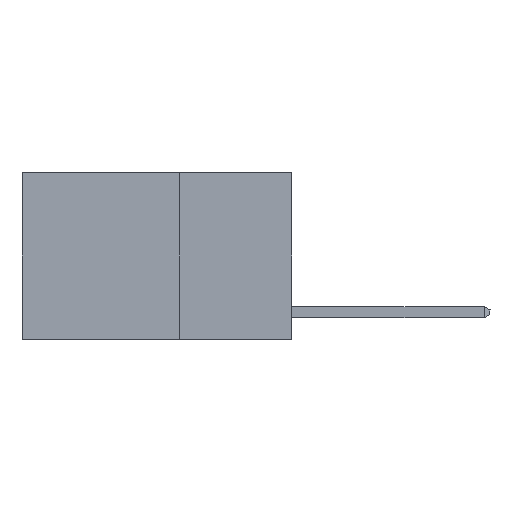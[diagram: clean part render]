
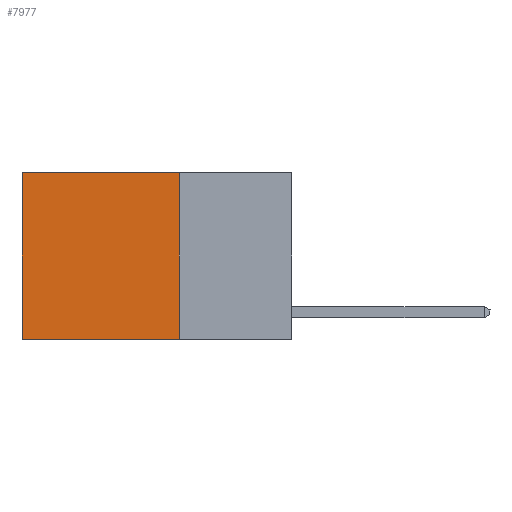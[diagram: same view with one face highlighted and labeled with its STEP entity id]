
A CAD part, left-side view. The second image highlights one B-rep face of the part: STEP entity #7977.
In plain terms, the highlighted planar face has unit normal (-1, 0, 0).
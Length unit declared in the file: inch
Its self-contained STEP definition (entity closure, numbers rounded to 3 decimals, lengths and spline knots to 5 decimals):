
#312 = LINE ( 'NONE', #19547, #20557 ) ;
#1221 = VERTEX_POINT ( 'NONE', #10538 ) ;
#2257 = LINE ( 'NONE', #14778, #7139 ) ;
#2525 = PLANE ( 'NONE',  #7700 ) ;
#3146 = CARTESIAN_POINT ( 'NONE',  ( 0.2625, 0.6, 0. ) ) ;
#3220 = DIRECTION ( 'NONE',  ( 0., 0., -1. ) ) ;
#3343 = DIRECTION ( 'NONE',  ( 0., 0., -1. ) ) ;
#5837 = DIRECTION ( 'NONE',  ( 0., 0., -1. ) ) ;
#6617 = CARTESIAN_POINT ( 'NONE',  ( 0.2625, 0.25, 0. ) ) ;
#7135 = VERTEX_POINT ( 'NONE', #11772 ) ;
#7139 = VECTOR ( 'NONE', #3343, 39.37008 ) ;
#7265 = DIRECTION ( 'NONE',  ( 0., 1., 0. ) ) ;
#7700 = AXIS2_PLACEMENT_3D ( 'NONE', #13976, #15629, #5837 ) ;
#7977 = ADVANCED_FACE ( 'NONE', ( #11208 ), #2525, .F. ) ;
#9650 = CARTESIAN_POINT ( 'NONE',  ( 0.2625, 0.25, -0.37 ) ) ;
#9879 = EDGE_CURVE ( 'NONE', #1221, #7135, #12168, .T. ) ;
#10538 = CARTESIAN_POINT ( 'NONE',  ( 0.2625, 0.25, -0.37 ) ) ;
#11208 = FACE_OUTER_BOUND ( 'NONE', #18272, .T. ) ;
#11658 = VECTOR ( 'NONE', #14513, 39.37008 ) ;
#11772 = CARTESIAN_POINT ( 'NONE',  ( 0.2625, 0.6, -0.37 ) ) ;
#12168 = LINE ( 'NONE', #9650, #11658 ) ;
#12485 = ORIENTED_EDGE ( 'NONE', *, *, #19044, .T. ) ;
#12974 = LINE ( 'NONE', #17092, #17347 ) ;
#13976 = CARTESIAN_POINT ( 'NONE',  ( 0.2625, 0.25, 0. ) ) ;
#14500 = VERTEX_POINT ( 'NONE', #6617 ) ;
#14513 = DIRECTION ( 'NONE',  ( 0., 1., 0. ) ) ;
#14778 = CARTESIAN_POINT ( 'NONE',  ( 0.2625, 0.6, 0. ) ) ;
#15321 = VERTEX_POINT ( 'NONE', #3146 ) ;
#15340 = EDGE_CURVE ( 'NONE', #14500, #1221, #312, .T. ) ;
#15629 = DIRECTION ( 'NONE',  ( 1., 0., 0. ) ) ;
#16818 = ORIENTED_EDGE ( 'NONE', *, *, #15340, .F. ) ;
#17092 = CARTESIAN_POINT ( 'NONE',  ( 0.2625, 0.25, 0. ) ) ;
#17347 = VECTOR ( 'NONE', #7265, 39.37008 ) ;
#17406 = ORIENTED_EDGE ( 'NONE', *, *, #17868, .T. ) ;
#17868 = EDGE_CURVE ( 'NONE', #15321, #7135, #2257, .T. ) ;
#18272 = EDGE_LOOP ( 'NONE', ( #17406, #19091, #16818, #12485 ) ) ;
#19044 = EDGE_CURVE ( 'NONE', #14500, #15321, #12974, .T. ) ;
#19091 = ORIENTED_EDGE ( 'NONE', *, *, #9879, .F. ) ;
#19547 = CARTESIAN_POINT ( 'NONE',  ( 0.2625, 0.25, 0. ) ) ;
#20557 = VECTOR ( 'NONE', #3220, 39.37008 ) ;
